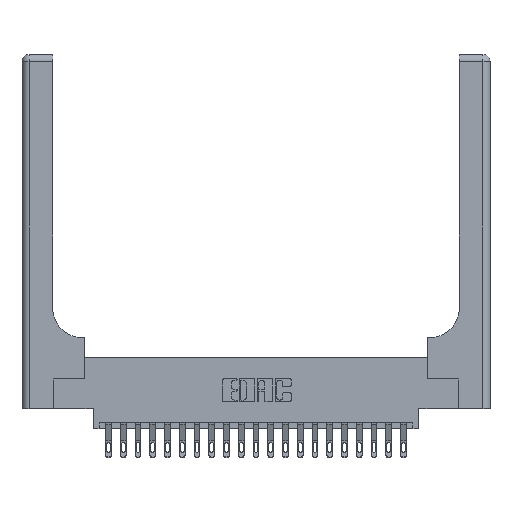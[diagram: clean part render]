
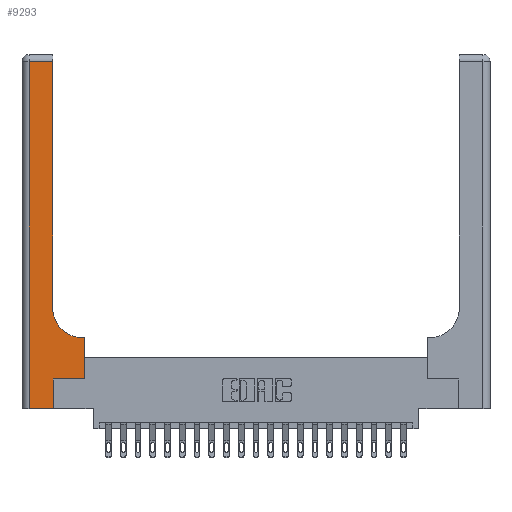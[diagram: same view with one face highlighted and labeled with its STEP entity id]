
A CAD part, top view. The second image highlights one B-rep face of the part: STEP entity #9293.
In plain terms, the highlighted planar face has unit normal (0, 0, 1).
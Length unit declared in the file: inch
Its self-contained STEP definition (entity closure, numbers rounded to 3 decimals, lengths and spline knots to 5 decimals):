
#2 = EDGE_LOOP ( 'NONE', ( #15955, #12532, #14032, #13194, #19033, #14123, #10739, #8140, #15547 ) ) ;
#60 = VERTEX_POINT ( 'NONE', #12857 ) ;
#369 = CARTESIAN_POINT ( 'NONE',  ( 0.06, 2.94, 0.37 ) ) ;
#737 = CARTESIAN_POINT ( 'NONE',  ( 0., 3., 0.37 ) ) ;
#952 = CARTESIAN_POINT ( 'NONE',  ( 0.06, 3., 0.37 ) ) ;
#1381 = VECTOR ( 'NONE', #5230, 39.37008 ) ;
#1903 = CARTESIAN_POINT ( 'NONE',  ( 0.51, 0.6, 0.37 ) ) ;
#3426 = VERTEX_POINT ( 'NONE', #1903 ) ;
#3677 = VERTEX_POINT ( 'NONE', #17944 ) ;
#4162 = LINE ( 'NONE', #6383, #21793 ) ;
#4612 = EDGE_CURVE ( 'NONE', #7210, #60, #14806, .T. ) ;
#5001 = CARTESIAN_POINT ( 'NONE',  ( 0.51, 0.85, 0.37 ) ) ;
#5230 = DIRECTION ( 'NONE',  ( -1., 0., 0. ) ) ;
#5287 = VECTOR ( 'NONE', #21252, 39.37008 ) ;
#5395 = CARTESIAN_POINT ( 'NONE',  ( 0.528, 0.6, 0.37 ) ) ;
#5633 = LINE ( 'NONE', #16952, #13650 ) ;
#5837 = EDGE_CURVE ( 'NONE', #3426, #13372, #10462, .T. ) ;
#6383 = CARTESIAN_POINT ( 'NONE',  ( 0.26, 3., 0.37 ) ) ;
#6586 = VECTOR ( 'NONE', #16906, 39.37008 ) ;
#6713 = CARTESIAN_POINT ( 'NONE',  ( 0.265, 0.25, 0.37 ) ) ;
#6747 = DIRECTION ( 'NONE',  ( 1., 0., 0. ) ) ;
#7210 = VERTEX_POINT ( 'NONE', #21834 ) ;
#7340 = CARTESIAN_POINT ( 'NONE',  ( 0.06, 0., 0.37 ) ) ;
#7653 = VECTOR ( 'NONE', #10784, 39.37008 ) ;
#7707 = DIRECTION ( 'NONE',  ( -1., 0., 0. ) ) ;
#8140 = ORIENTED_EDGE ( 'NONE', *, *, #10584, .T. ) ;
#8613 = DIRECTION ( 'NONE',  ( 0., 1., 0. ) ) ;
#8825 = EDGE_CURVE ( 'NONE', #10745, #3677, #15678, .T. ) ;
#9060 = CARTESIAN_POINT ( 'NONE',  ( 0.26, 0.6, 0.37 ) ) ;
#9116 = VERTEX_POINT ( 'NONE', #369 ) ;
#9293 = ADVANCED_FACE ( 'NONE', ( #15655 ), #16226, .F. ) ;
#10187 = CARTESIAN_POINT ( 'NONE',  ( 0.528, 0.25, 0.37 ) ) ;
#10271 = VERTEX_POINT ( 'NONE', #11246 ) ;
#10462 = CIRCLE ( 'NONE', #14067, 0.25 ) ;
#10584 = EDGE_CURVE ( 'NONE', #14543, #3426, #11618, .T. ) ;
#10739 = ORIENTED_EDGE ( 'NONE', *, *, #14953, .T. ) ;
#10745 = VERTEX_POINT ( 'NONE', #7340 ) ;
#10784 = DIRECTION ( 'NONE',  ( 0., -1., 0. ) ) ;
#11246 = CARTESIAN_POINT ( 'NONE',  ( 0.26, 2.94, 0.37 ) ) ;
#11548 = EDGE_CURVE ( 'NONE', #9116, #10745, #16731, .T. ) ;
#11618 = LINE ( 'NONE', #9060, #1381 ) ;
#12532 = ORIENTED_EDGE ( 'NONE', *, *, #17286, .T. ) ;
#12699 = CARTESIAN_POINT ( 'NONE',  ( 0., 2.94, 0.37 ) ) ;
#12857 = CARTESIAN_POINT ( 'NONE',  ( 0.528, 0.25, 0.37 ) ) ;
#12894 = VECTOR ( 'NONE', #8613, 39.37008 ) ;
#13194 = ORIENTED_EDGE ( 'NONE', *, *, #8825, .T. ) ;
#13372 = VERTEX_POINT ( 'NONE', #21067 ) ;
#13650 = VECTOR ( 'NONE', #18660, 39.37008 ) ;
#14032 = ORIENTED_EDGE ( 'NONE', *, *, #11548, .T. ) ;
#14067 = AXIS2_PLACEMENT_3D ( 'NONE', #5001, #16984, #6747 ) ;
#14123 = ORIENTED_EDGE ( 'NONE', *, *, #4612, .T. ) ;
#14411 = LINE ( 'NONE', #12699, #5287 ) ;
#14543 = VERTEX_POINT ( 'NONE', #5395 ) ;
#14806 = LINE ( 'NONE', #6713, #18793 ) ;
#14953 = EDGE_CURVE ( 'NONE', #60, #14543, #17436, .T. ) ;
#15214 = CARTESIAN_POINT ( 'NONE',  ( 0., 0., 0.37 ) ) ;
#15547 = ORIENTED_EDGE ( 'NONE', *, *, #5837, .T. ) ;
#15655 = FACE_OUTER_BOUND ( 'NONE', #2, .T. ) ;
#15678 = LINE ( 'NONE', #15214, #6586 ) ;
#15955 = ORIENTED_EDGE ( 'NONE', *, *, #21139, .T. ) ;
#16226 = PLANE ( 'NONE',  #17808 ) ;
#16600 = DIRECTION ( 'NONE',  ( 0., 1., 0. ) ) ;
#16731 = LINE ( 'NONE', #952, #7653 ) ;
#16906 = DIRECTION ( 'NONE',  ( 1., 0., 0. ) ) ;
#16952 = CARTESIAN_POINT ( 'NONE',  ( 0.265, 0., 0.37 ) ) ;
#16984 = DIRECTION ( 'NONE',  ( 0., 0., -1. ) ) ;
#17286 = EDGE_CURVE ( 'NONE', #10271, #9116, #14411, .T. ) ;
#17436 = LINE ( 'NONE', #10187, #12894 ) ;
#17808 = AXIS2_PLACEMENT_3D ( 'NONE', #737, #17930, #7707 ) ;
#17930 = DIRECTION ( 'NONE',  ( 0., 0., -1. ) ) ;
#17944 = CARTESIAN_POINT ( 'NONE',  ( 0.265, 0., 0.37 ) ) ;
#18654 = DIRECTION ( 'NONE',  ( 1., 0., 0. ) ) ;
#18660 = DIRECTION ( 'NONE',  ( 0., 1., 0. ) ) ;
#18793 = VECTOR ( 'NONE', #18654, 39.37008 ) ;
#18948 = EDGE_CURVE ( 'NONE', #3677, #7210, #5633, .T. ) ;
#19033 = ORIENTED_EDGE ( 'NONE', *, *, #18948, .T. ) ;
#21067 = CARTESIAN_POINT ( 'NONE',  ( 0.26, 0.85, 0.37 ) ) ;
#21139 = EDGE_CURVE ( 'NONE', #13372, #10271, #4162, .T. ) ;
#21252 = DIRECTION ( 'NONE',  ( -1., 0., 0. ) ) ;
#21793 = VECTOR ( 'NONE', #16600, 39.37008 ) ;
#21834 = CARTESIAN_POINT ( 'NONE',  ( 0.265, 0.25, 0.37 ) ) ;
